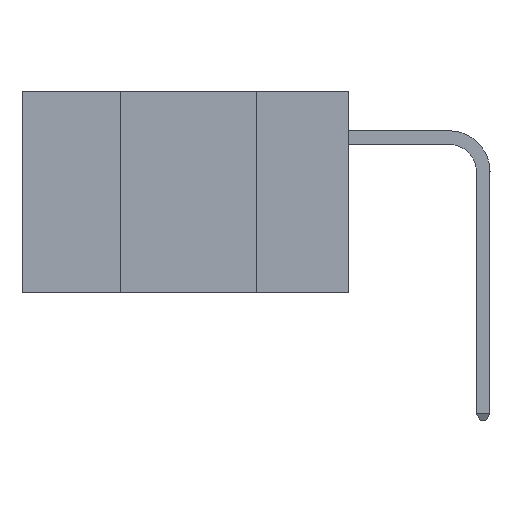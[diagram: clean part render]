
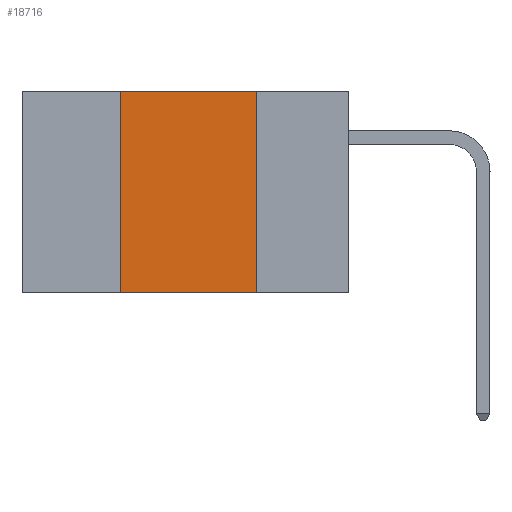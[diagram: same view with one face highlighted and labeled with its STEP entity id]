
A CAD part, left-side view. The second image highlights one B-rep face of the part: STEP entity #18716.
In plain terms, the highlighted planar face has unit normal (-1, 0, 0).
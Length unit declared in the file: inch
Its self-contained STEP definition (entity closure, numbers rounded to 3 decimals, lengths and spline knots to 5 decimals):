
#41 = LINE ( 'NONE', #5161, #6532 ) ;
#1193 = CARTESIAN_POINT ( 'NONE',  ( 0., 0.42, -0.37 ) ) ;
#1633 = VECTOR ( 'NONE', #2077, 39.37008 ) ;
#2077 = DIRECTION ( 'NONE',  ( 0., 0., -1. ) ) ;
#2886 = VERTEX_POINT ( 'NONE', #1193 ) ;
#3090 = ORIENTED_EDGE ( 'NONE', *, *, #14222, .T. ) ;
#3437 = ORIENTED_EDGE ( 'NONE', *, *, #16471, .F. ) ;
#3625 = LINE ( 'NONE', #19329, #1633 ) ;
#3636 = ORIENTED_EDGE ( 'NONE', *, *, #3847, .F. ) ;
#3847 = EDGE_CURVE ( 'NONE', #15191, #12855, #3625, .T. ) ;
#3911 = FACE_OUTER_BOUND ( 'NONE', #8453, .T. ) ;
#5161 = CARTESIAN_POINT ( 'NONE',  ( 0., 0.6, 0. ) ) ;
#5471 = DIRECTION ( 'NONE',  ( 1., 0., 0. ) ) ;
#5524 = CARTESIAN_POINT ( 'NONE',  ( 0., 0.17, -0.37 ) ) ;
#6532 = VECTOR ( 'NONE', #9969, 39.37008 ) ;
#6924 = CARTESIAN_POINT ( 'NONE',  ( 0., 0.42, 0. ) ) ;
#7396 = EDGE_CURVE ( 'NONE', #2886, #13098, #17694, .T. ) ;
#8453 = EDGE_LOOP ( 'NONE', ( #3636, #3437, #9085, #3090 ) ) ;
#9085 = ORIENTED_EDGE ( 'NONE', *, *, #7396, .F. ) ;
#9786 = DIRECTION ( 'NONE',  ( 0., -1., 0. ) ) ;
#9969 = DIRECTION ( 'NONE',  ( 0., -1., 0. ) ) ;
#11658 = CARTESIAN_POINT ( 'NONE',  ( 0., 0.42, 0. ) ) ;
#12855 = VERTEX_POINT ( 'NONE', #5524 ) ;
#13098 = VERTEX_POINT ( 'NONE', #6924 ) ;
#14039 = CARTESIAN_POINT ( 'NONE',  ( 0., 0.17, 0. ) ) ;
#14222 = EDGE_CURVE ( 'NONE', #2886, #12855, #17512, .T. ) ;
#14874 = DIRECTION ( 'NONE',  ( 0., 0., 1. ) ) ;
#15191 = VERTEX_POINT ( 'NONE', #14039 ) ;
#16288 = AXIS2_PLACEMENT_3D ( 'NONE', #16746, #5471, #19705 ) ;
#16471 = EDGE_CURVE ( 'NONE', #13098, #15191, #41, .T. ) ;
#16618 = PLANE ( 'NONE',  #16288 ) ;
#16746 = CARTESIAN_POINT ( 'NONE',  ( 0., 0.6, 0. ) ) ;
#17512 = LINE ( 'NONE', #17716, #19286 ) ;
#17673 = VECTOR ( 'NONE', #14874, 39.37008 ) ;
#17694 = LINE ( 'NONE', #11658, #17673 ) ;
#17716 = CARTESIAN_POINT ( 'NONE',  ( 0., 0.6, -0.37 ) ) ;
#18716 = ADVANCED_FACE ( 'NONE', ( #3911 ), #16618, .F. ) ;
#19286 = VECTOR ( 'NONE', #9786, 39.37008 ) ;
#19329 = CARTESIAN_POINT ( 'NONE',  ( 0., 0.17, 0. ) ) ;
#19705 = DIRECTION ( 'NONE',  ( 0., 0., -1. ) ) ;
